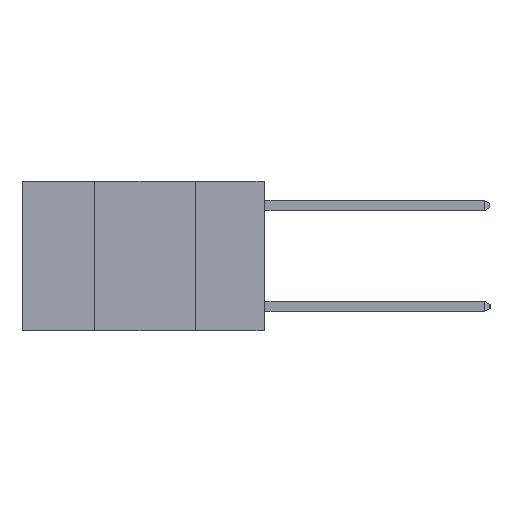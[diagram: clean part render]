
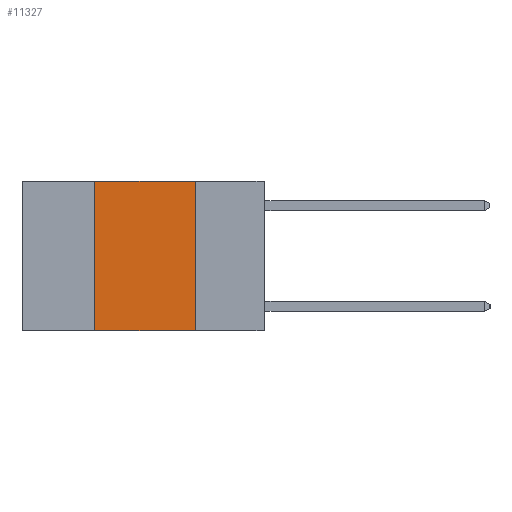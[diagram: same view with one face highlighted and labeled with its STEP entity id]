
A CAD part, left-side view. The second image highlights one B-rep face of the part: STEP entity #11327.
In plain terms, the highlighted planar face has unit normal (-1, 0, 0).
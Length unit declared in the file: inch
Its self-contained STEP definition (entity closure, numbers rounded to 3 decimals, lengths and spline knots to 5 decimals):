
#722 = VERTEX_POINT ( 'NONE', #9141 ) ;
#1221 = DIRECTION ( 'NONE',  ( 0., 0., 1. ) ) ;
#1321 = ORIENTED_EDGE ( 'NONE', *, *, #9107, .F. ) ;
#1509 = CARTESIAN_POINT ( 'NONE',  ( 0., 0.17, 0. ) ) ;
#1514 = LINE ( 'NONE', #11708, #3679 ) ;
#1670 = VECTOR ( 'NONE', #1221, 39.37008 ) ;
#1900 = DIRECTION ( 'NONE',  ( 0., 0., -1. ) ) ;
#2493 = FACE_OUTER_BOUND ( 'NONE', #7030, .T. ) ;
#3195 = DIRECTION ( 'NONE',  ( 0., -1., 0. ) ) ;
#3493 = DIRECTION ( 'NONE',  ( 0., -1., 0. ) ) ;
#3679 = VECTOR ( 'NONE', #3493, 39.37008 ) ;
#3821 = LINE ( 'NONE', #9614, #10572 ) ;
#4565 = VECTOR ( 'NONE', #5493, 39.37008 ) ;
#5368 = VERTEX_POINT ( 'NONE', #1509 ) ;
#5493 = DIRECTION ( 'NONE',  ( 0., 0., -1. ) ) ;
#5634 = ORIENTED_EDGE ( 'NONE', *, *, #9326, .F. ) ;
#5637 = AXIS2_PLACEMENT_3D ( 'NONE', #8304, #7414, #1900 ) ;
#6189 = ORIENTED_EDGE ( 'NONE', *, *, #8744, .T. ) ;
#7030 = EDGE_LOOP ( 'NONE', ( #1321, #10647, #5634, #6189 ) ) ;
#7414 = DIRECTION ( 'NONE',  ( 1., 0., 0. ) ) ;
#7991 = VERTEX_POINT ( 'NONE', #11812 ) ;
#8304 = CARTESIAN_POINT ( 'NONE',  ( 0., 0.6, 0. ) ) ;
#8606 = CARTESIAN_POINT ( 'NONE',  ( 0., 0.42, 0. ) ) ;
#8744 = EDGE_CURVE ( 'NONE', #7991, #9587, #3821, .T. ) ;
#8986 = CARTESIAN_POINT ( 'NONE',  ( 0., 0.17, -0.37 ) ) ;
#8993 = LINE ( 'NONE', #8606, #1670 ) ;
#9107 = EDGE_CURVE ( 'NONE', #5368, #9587, #11849, .T. ) ;
#9141 = CARTESIAN_POINT ( 'NONE',  ( 0., 0.42, 0. ) ) ;
#9326 = EDGE_CURVE ( 'NONE', #7991, #722, #8993, .T. ) ;
#9585 = EDGE_CURVE ( 'NONE', #722, #5368, #1514, .T. ) ;
#9587 = VERTEX_POINT ( 'NONE', #8986 ) ;
#9614 = CARTESIAN_POINT ( 'NONE',  ( 0., 0.6, -0.37 ) ) ;
#10572 = VECTOR ( 'NONE', #3195, 39.37008 ) ;
#10647 = ORIENTED_EDGE ( 'NONE', *, *, #9585, .F. ) ;
#11066 = PLANE ( 'NONE',  #5637 ) ;
#11327 = ADVANCED_FACE ( 'NONE', ( #2493 ), #11066, .F. ) ;
#11708 = CARTESIAN_POINT ( 'NONE',  ( 0., 0.6, 0. ) ) ;
#11812 = CARTESIAN_POINT ( 'NONE',  ( 0., 0.42, -0.37 ) ) ;
#11849 = LINE ( 'NONE', #11865, #4565 ) ;
#11865 = CARTESIAN_POINT ( 'NONE',  ( 0., 0.17, 0. ) ) ;
